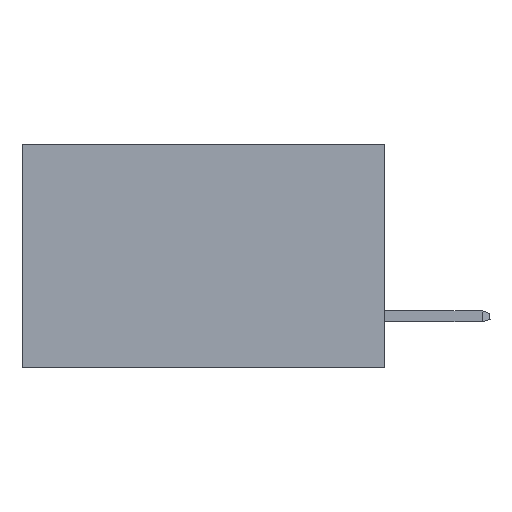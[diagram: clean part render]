
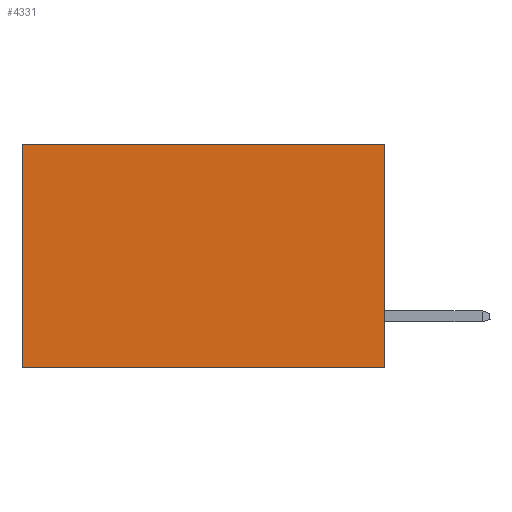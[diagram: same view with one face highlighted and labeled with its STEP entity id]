
A CAD part, left-side view. The second image highlights one B-rep face of the part: STEP entity #4331.
In plain terms, the highlighted planar face has unit normal (-1, 0, 0).
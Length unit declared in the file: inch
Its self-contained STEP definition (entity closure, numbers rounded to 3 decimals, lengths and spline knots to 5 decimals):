
#1533 = DIRECTION ( 'NONE',  ( 0., 0., -1. ) ) ;
#2744 = ORIENTED_EDGE ( 'NONE', *, *, #24166, .F. ) ;
#3151 = EDGE_LOOP ( 'NONE', ( #25087, #12199, #2744, #24985 ) ) ;
#3152 = LINE ( 'NONE', #8416, #24975 ) ;
#4224 = DIRECTION ( 'NONE',  ( 0., 1., 0. ) ) ;
#4331 = ADVANCED_FACE ( 'NONE', ( #18817 ), #24117, .F. ) ;
#5627 = LINE ( 'NONE', #19667, #21426 ) ;
#5900 = VERTEX_POINT ( 'NONE', #6813 ) ;
#6723 = DIRECTION ( 'NONE',  ( 0., 0., -1. ) ) ;
#6813 = CARTESIAN_POINT ( 'NONE',  ( 0.298, 0.6, 0. ) ) ;
#8289 = CARTESIAN_POINT ( 'NONE',  ( 0.298, 0., -0.37 ) ) ;
#8416 = CARTESIAN_POINT ( 'NONE',  ( 0.298, 0.6, 0. ) ) ;
#8789 = AXIS2_PLACEMENT_3D ( 'NONE', #21958, #28847, #17339 ) ;
#10667 = DIRECTION ( 'NONE',  ( 0., 1., 0. ) ) ;
#12199 = ORIENTED_EDGE ( 'NONE', *, *, #17922, .F. ) ;
#14070 = VERTEX_POINT ( 'NONE', #26589 ) ;
#15498 = CARTESIAN_POINT ( 'NONE',  ( 0.298, 0., 0. ) ) ;
#15850 = CARTESIAN_POINT ( 'NONE',  ( 0.298, 0., 0. ) ) ;
#17339 = DIRECTION ( 'NONE',  ( 0., 0., -1. ) ) ;
#17562 = LINE ( 'NONE', #15850, #19317 ) ;
#17892 = EDGE_CURVE ( 'NONE', #5900, #14070, #3152, .T. ) ;
#17922 = EDGE_CURVE ( 'NONE', #22271, #14070, #5627, .T. ) ;
#18817 = FACE_OUTER_BOUND ( 'NONE', #3151, .T. ) ;
#19317 = VECTOR ( 'NONE', #6723, 39.37008 ) ;
#19667 = CARTESIAN_POINT ( 'NONE',  ( 0.298, 0., -0.37 ) ) ;
#20147 = EDGE_CURVE ( 'NONE', #24612, #5900, #25786, .T. ) ;
#20876 = VECTOR ( 'NONE', #4224, 39.37008 ) ;
#21426 = VECTOR ( 'NONE', #10667, 39.37008 ) ;
#21958 = CARTESIAN_POINT ( 'NONE',  ( 0.298, 0., 0. ) ) ;
#22271 = VERTEX_POINT ( 'NONE', #8289 ) ;
#22322 = CARTESIAN_POINT ( 'NONE',  ( 0.298, 0., 0. ) ) ;
#24117 = PLANE ( 'NONE',  #8789 ) ;
#24166 = EDGE_CURVE ( 'NONE', #24612, #22271, #17562, .T. ) ;
#24612 = VERTEX_POINT ( 'NONE', #22322 ) ;
#24975 = VECTOR ( 'NONE', #1533, 39.37008 ) ;
#24985 = ORIENTED_EDGE ( 'NONE', *, *, #20147, .T. ) ;
#25087 = ORIENTED_EDGE ( 'NONE', *, *, #17892, .T. ) ;
#25786 = LINE ( 'NONE', #15498, #20876 ) ;
#26589 = CARTESIAN_POINT ( 'NONE',  ( 0.298, 0.6, -0.37 ) ) ;
#28847 = DIRECTION ( 'NONE',  ( 1., 0., 0. ) ) ;
